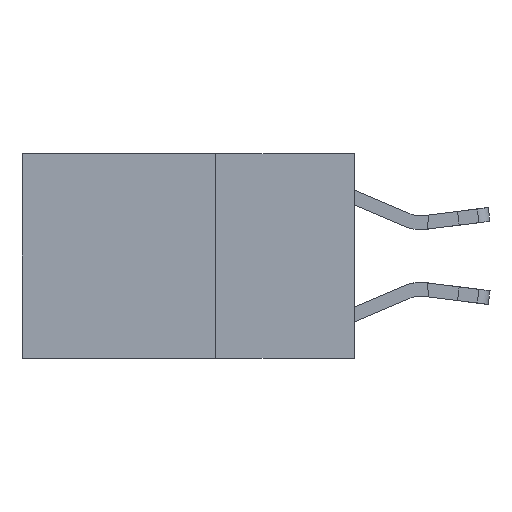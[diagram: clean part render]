
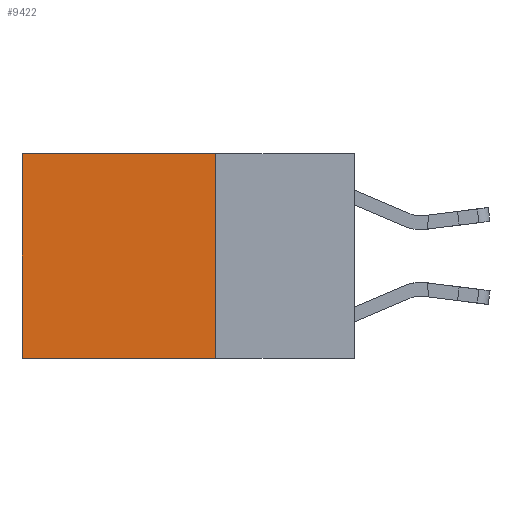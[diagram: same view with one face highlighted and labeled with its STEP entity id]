
A CAD part, left-side view. The second image highlights one B-rep face of the part: STEP entity #9422.
In plain terms, the highlighted planar face has unit normal (-1, 0, 0).
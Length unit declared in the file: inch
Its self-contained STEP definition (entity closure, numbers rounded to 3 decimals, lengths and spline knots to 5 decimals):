
#249 = LINE ( 'NONE', #12855, #6456 ) ;
#409 = CARTESIAN_POINT ( 'NONE',  ( 0.2625, 0.25, 0. ) ) ;
#1704 = ORIENTED_EDGE ( 'NONE', *, *, #15623, .F. ) ;
#1779 = DIRECTION ( 'NONE',  ( 0., 1., 0. ) ) ;
#1913 = VERTEX_POINT ( 'NONE', #15773 ) ;
#2802 = ORIENTED_EDGE ( 'NONE', *, *, #12967, .T. ) ;
#2951 = EDGE_CURVE ( 'NONE', #4827, #11640, #5614, .T. ) ;
#3230 = DIRECTION ( 'NONE',  ( 0., 1., 0. ) ) ;
#3404 = EDGE_LOOP ( 'NONE', ( #9886, #1704, #15010, #2802 ) ) ;
#3570 = AXIS2_PLACEMENT_3D ( 'NONE', #12516, #6359, #14982 ) ;
#3885 = PLANE ( 'NONE',  #3570 ) ;
#4163 = DIRECTION ( 'NONE',  ( 0., 0., -1. ) ) ;
#4681 = VECTOR ( 'NONE', #1779, 39.37008 ) ;
#4827 = VERTEX_POINT ( 'NONE', #9329 ) ;
#5504 = LINE ( 'NONE', #10625, #11693 ) ;
#5614 = LINE ( 'NONE', #409, #8540 ) ;
#6359 = DIRECTION ( 'NONE',  ( 1., 0., 0. ) ) ;
#6456 = VECTOR ( 'NONE', #11673, 39.37008 ) ;
#8540 = VECTOR ( 'NONE', #4163, 39.37008 ) ;
#9329 = CARTESIAN_POINT ( 'NONE',  ( 0.2625, 0.25, 0. ) ) ;
#9422 = ADVANCED_FACE ( 'NONE', ( #15566 ), #3885, .F. ) ;
#9886 = ORIENTED_EDGE ( 'NONE', *, *, #15532, .T. ) ;
#10402 = CARTESIAN_POINT ( 'NONE',  ( 0.2625, 0.25, 0. ) ) ;
#10625 = CARTESIAN_POINT ( 'NONE',  ( 0.2625, 0.25, -0.37 ) ) ;
#11225 = LINE ( 'NONE', #10402, #4681 ) ;
#11640 = VERTEX_POINT ( 'NONE', #11747 ) ;
#11673 = DIRECTION ( 'NONE',  ( 0., 0., -1. ) ) ;
#11693 = VECTOR ( 'NONE', #3230, 39.37008 ) ;
#11747 = CARTESIAN_POINT ( 'NONE',  ( 0.2625, 0.25, -0.37 ) ) ;
#12516 = CARTESIAN_POINT ( 'NONE',  ( 0.2625, 0.25, 0. ) ) ;
#12855 = CARTESIAN_POINT ( 'NONE',  ( 0.2625, 0.6, 0. ) ) ;
#12967 = EDGE_CURVE ( 'NONE', #4827, #1913, #11225, .T. ) ;
#13914 = CARTESIAN_POINT ( 'NONE',  ( 0.2625, 0.6, -0.37 ) ) ;
#14084 = VERTEX_POINT ( 'NONE', #13914 ) ;
#14982 = DIRECTION ( 'NONE',  ( 0., 0., -1. ) ) ;
#15010 = ORIENTED_EDGE ( 'NONE', *, *, #2951, .F. ) ;
#15532 = EDGE_CURVE ( 'NONE', #1913, #14084, #249, .T. ) ;
#15566 = FACE_OUTER_BOUND ( 'NONE', #3404, .T. ) ;
#15623 = EDGE_CURVE ( 'NONE', #11640, #14084, #5504, .T. ) ;
#15773 = CARTESIAN_POINT ( 'NONE',  ( 0.2625, 0.6, 0. ) ) ;
